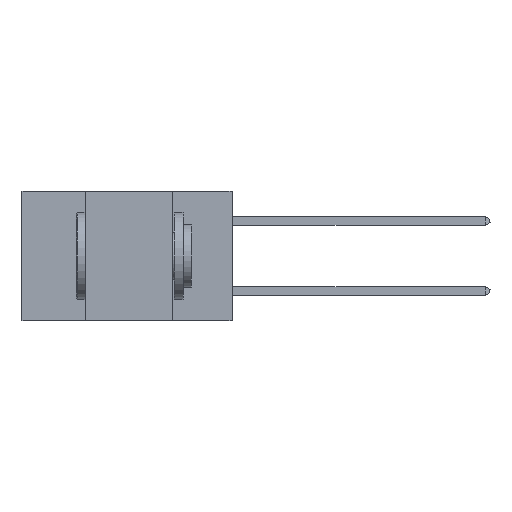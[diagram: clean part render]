
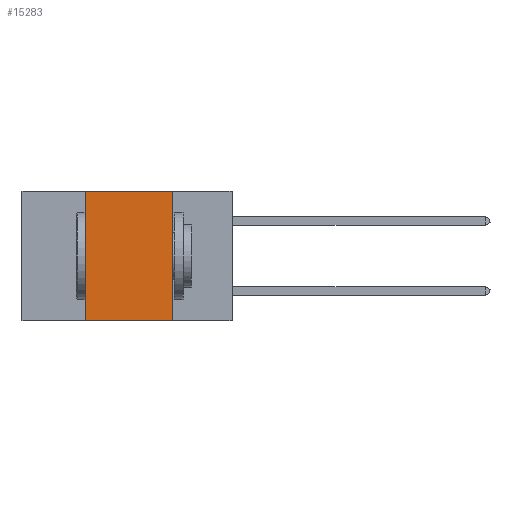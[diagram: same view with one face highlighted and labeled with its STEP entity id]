
A CAD part, left-side view. The second image highlights one B-rep face of the part: STEP entity #15283.
In plain terms, the highlighted planar face has unit normal (-1, 0, 0).
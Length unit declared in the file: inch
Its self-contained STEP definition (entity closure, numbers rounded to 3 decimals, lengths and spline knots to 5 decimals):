
#618 = VERTEX_POINT ( 'NONE', #21712 ) ;
#2070 = EDGE_CURVE ( 'NONE', #3877, #22801, #7076, .T. ) ;
#2798 = CARTESIAN_POINT ( 'NONE',  ( 0., 0.17, -0.37 ) ) ;
#3012 = CARTESIAN_POINT ( 'NONE',  ( 0., 0.6, 0. ) ) ;
#3877 = VERTEX_POINT ( 'NONE', #14271 ) ;
#4264 = VECTOR ( 'NONE', #19438, 39.37008 ) ;
#4627 = ORIENTED_EDGE ( 'NONE', *, *, #6468, .F. ) ;
#5276 = DIRECTION ( 'NONE',  ( 0., 0., -1. ) ) ;
#6468 = EDGE_CURVE ( 'NONE', #618, #11856, #11136, .T. ) ;
#7008 = PLANE ( 'NONE',  #18861 ) ;
#7076 = LINE ( 'NONE', #19598, #21522 ) ;
#7612 = DIRECTION ( 'NONE',  ( 0., 0., -1. ) ) ;
#8648 = ORIENTED_EDGE ( 'NONE', *, *, #13337, .F. ) ;
#11136 = LINE ( 'NONE', #18421, #15859 ) ;
#11856 = VERTEX_POINT ( 'NONE', #2798 ) ;
#11866 = ORIENTED_EDGE ( 'NONE', *, *, #16687, .T. ) ;
#12491 = CARTESIAN_POINT ( 'NONE',  ( 0., 0.6, 0. ) ) ;
#13337 = EDGE_CURVE ( 'NONE', #22801, #618, #22432, .T. ) ;
#14271 = CARTESIAN_POINT ( 'NONE',  ( 0., 0.42, -0.37 ) ) ;
#15283 = ADVANCED_FACE ( 'NONE', ( #17150 ), #7008, .F. ) ;
#15859 = VECTOR ( 'NONE', #7612, 39.37008 ) ;
#16042 = DIRECTION ( 'NONE',  ( 1., 0., 0. ) ) ;
#16687 = EDGE_CURVE ( 'NONE', #3877, #11856, #17403, .T. ) ;
#16825 = VECTOR ( 'NONE', #17091, 39.37008 ) ;
#17091 = DIRECTION ( 'NONE',  ( 0., -1., 0. ) ) ;
#17150 = FACE_OUTER_BOUND ( 'NONE', #21497, .T. ) ;
#17403 = LINE ( 'NONE', #20671, #16825 ) ;
#18421 = CARTESIAN_POINT ( 'NONE',  ( 0., 0.17, 0. ) ) ;
#18861 = AXIS2_PLACEMENT_3D ( 'NONE', #12491, #16042, #5276 ) ;
#19349 = DIRECTION ( 'NONE',  ( 0., 0., 1. ) ) ;
#19438 = DIRECTION ( 'NONE',  ( 0., -1., 0. ) ) ;
#19598 = CARTESIAN_POINT ( 'NONE',  ( 0., 0.42, 0. ) ) ;
#20671 = CARTESIAN_POINT ( 'NONE',  ( 0., 0.6, -0.37 ) ) ;
#21091 = ORIENTED_EDGE ( 'NONE', *, *, #2070, .F. ) ;
#21497 = EDGE_LOOP ( 'NONE', ( #4627, #8648, #21091, #11866 ) ) ;
#21522 = VECTOR ( 'NONE', #19349, 39.37008 ) ;
#21712 = CARTESIAN_POINT ( 'NONE',  ( 0., 0.17, 0. ) ) ;
#22124 = CARTESIAN_POINT ( 'NONE',  ( 0., 0.42, 0. ) ) ;
#22432 = LINE ( 'NONE', #3012, #4264 ) ;
#22801 = VERTEX_POINT ( 'NONE', #22124 ) ;
